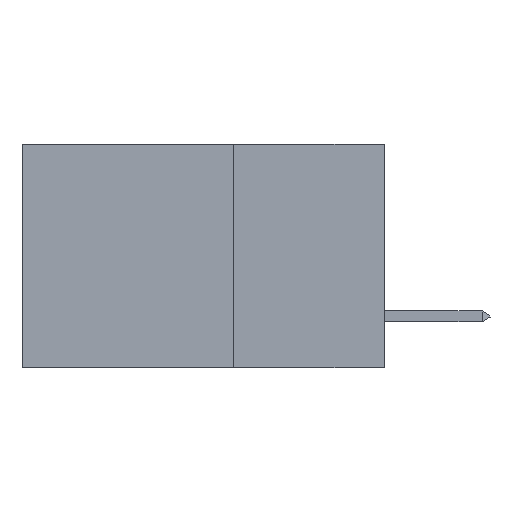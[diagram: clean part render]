
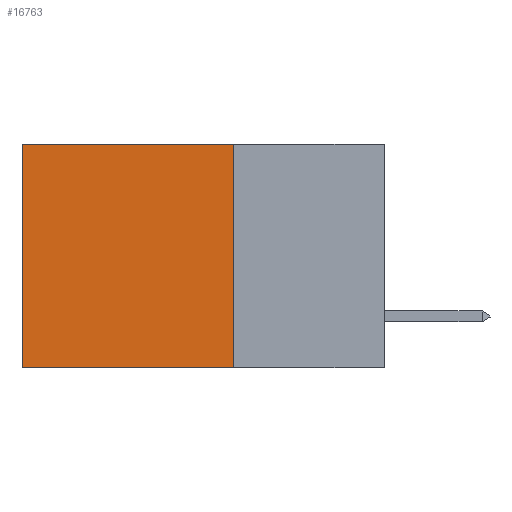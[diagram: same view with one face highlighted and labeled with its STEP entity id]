
A CAD part, left-side view. The second image highlights one B-rep face of the part: STEP entity #16763.
In plain terms, the highlighted planar face has unit normal (-1, 0, 0).
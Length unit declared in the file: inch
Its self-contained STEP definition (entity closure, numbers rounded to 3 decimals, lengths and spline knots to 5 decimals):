
#726 = LINE ( 'NONE', #3381, #10838 ) ;
#741 = CARTESIAN_POINT ( 'NONE',  ( 0.2875, 0.6, 0. ) ) ;
#836 = VECTOR ( 'NONE', #9614, 39.37008 ) ;
#1201 = CARTESIAN_POINT ( 'NONE',  ( 0.2875, 0.6, -0.37 ) ) ;
#1554 = CARTESIAN_POINT ( 'NONE',  ( 0.2875, 0.25, 0. ) ) ;
#2318 = ORIENTED_EDGE ( 'NONE', *, *, #11461, .T. ) ;
#2451 = DIRECTION ( 'NONE',  ( 0., 0., -1. ) ) ;
#2978 = DIRECTION ( 'NONE',  ( 0., 1., 0. ) ) ;
#3381 = CARTESIAN_POINT ( 'NONE',  ( 0.2875, 0.25, 0. ) ) ;
#3992 = CARTESIAN_POINT ( 'NONE',  ( 0.2875, 0.25, -0.37 ) ) ;
#4119 = CARTESIAN_POINT ( 'NONE',  ( 0.2875, 0.25, 0. ) ) ;
#5620 = DIRECTION ( 'NONE',  ( 0., 0., -1. ) ) ;
#6244 = VERTEX_POINT ( 'NONE', #1201 ) ;
#6984 = EDGE_CURVE ( 'NONE', #18540, #6244, #16437, .T. ) ;
#7056 = PLANE ( 'NONE',  #15030 ) ;
#8243 = DIRECTION ( 'NONE',  ( 0., 0., -1. ) ) ;
#9119 = FACE_OUTER_BOUND ( 'NONE', #16619, .T. ) ;
#9215 = VERTEX_POINT ( 'NONE', #11102 ) ;
#9614 = DIRECTION ( 'NONE',  ( 0., 1., 0. ) ) ;
#9635 = VECTOR ( 'NONE', #5620, 39.37008 ) ;
#9763 = CARTESIAN_POINT ( 'NONE',  ( 0.2875, 0.6, 0. ) ) ;
#9806 = DIRECTION ( 'NONE',  ( 1., 0., 0. ) ) ;
#10685 = EDGE_CURVE ( 'NONE', #9215, #6244, #18431, .T. ) ;
#10838 = VECTOR ( 'NONE', #2451, 39.37008 ) ;
#11102 = CARTESIAN_POINT ( 'NONE',  ( 0.2875, 0.25, -0.37 ) ) ;
#11461 = EDGE_CURVE ( 'NONE', #13017, #18540, #18389, .T. ) ;
#11805 = VECTOR ( 'NONE', #2978, 39.37008 ) ;
#13017 = VERTEX_POINT ( 'NONE', #14391 ) ;
#13764 = EDGE_CURVE ( 'NONE', #13017, #9215, #726, .T. ) ;
#14257 = ORIENTED_EDGE ( 'NONE', *, *, #10685, .F. ) ;
#14391 = CARTESIAN_POINT ( 'NONE',  ( 0.2875, 0.25, 0. ) ) ;
#15030 = AXIS2_PLACEMENT_3D ( 'NONE', #4119, #9806, #8243 ) ;
#16437 = LINE ( 'NONE', #9763, #9635 ) ;
#16619 = EDGE_LOOP ( 'NONE', ( #18684, #14257, #18652, #2318 ) ) ;
#16763 = ADVANCED_FACE ( 'NONE', ( #9119 ), #7056, .F. ) ;
#18389 = LINE ( 'NONE', #1554, #11805 ) ;
#18431 = LINE ( 'NONE', #3992, #836 ) ;
#18540 = VERTEX_POINT ( 'NONE', #741 ) ;
#18652 = ORIENTED_EDGE ( 'NONE', *, *, #13764, .F. ) ;
#18684 = ORIENTED_EDGE ( 'NONE', *, *, #6984, .T. ) ;
